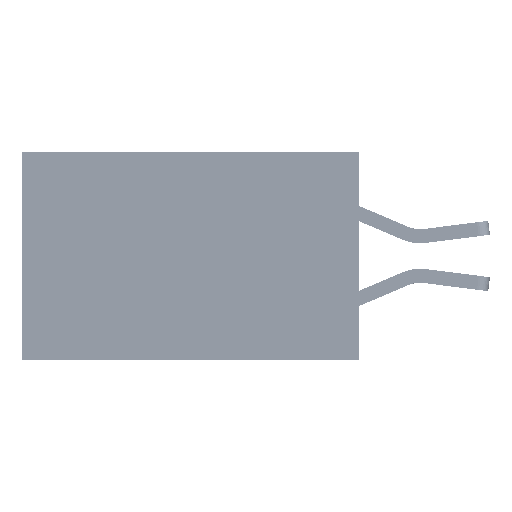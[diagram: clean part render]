
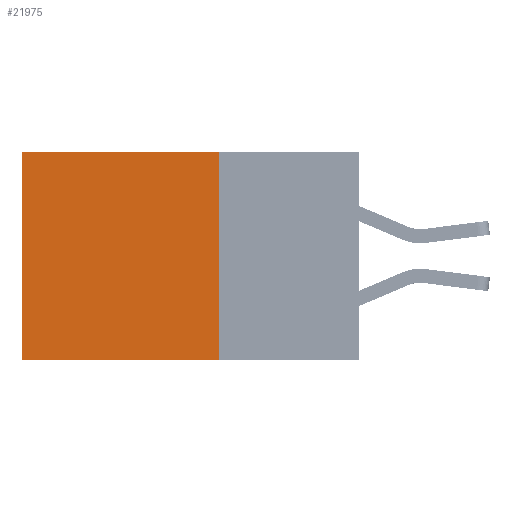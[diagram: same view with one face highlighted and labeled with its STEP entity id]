
A CAD part, left-side view. The second image highlights one B-rep face of the part: STEP entity #21975.
In plain terms, the highlighted planar face has unit normal (-1, 0, 0).
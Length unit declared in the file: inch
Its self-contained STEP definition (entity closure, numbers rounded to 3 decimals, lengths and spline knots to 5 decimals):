
#781 = DIRECTION ( 'NONE',  ( 0., 0., -1. ) ) ;
#990 = CARTESIAN_POINT ( 'NONE',  ( 0.2875, 0.25, -0.37 ) ) ;
#1263 = PLANE ( 'NONE',  #16572 ) ;
#1354 = ORIENTED_EDGE ( 'NONE', *, *, #22394, .T. ) ;
#1363 = LINE ( 'NONE', #17953, #22209 ) ;
#2689 = VERTEX_POINT ( 'NONE', #40871 ) ;
#2966 = DIRECTION ( 'NONE',  ( 0., 0., -1. ) ) ;
#4095 = ORIENTED_EDGE ( 'NONE', *, *, #32219, .T. ) ;
#7632 = CARTESIAN_POINT ( 'NONE',  ( 0.2875, 0.25, 0. ) ) ;
#13044 = ORIENTED_EDGE ( 'NONE', *, *, #46236, .F. ) ;
#14273 = CARTESIAN_POINT ( 'NONE',  ( 0.2875, 0.25, -0.37 ) ) ;
#15764 = CARTESIAN_POINT ( 'NONE',  ( 0.2875, 0.25, 0. ) ) ;
#16572 = AXIS2_PLACEMENT_3D ( 'NONE', #15764, #19606, #781 ) ;
#16774 = VECTOR ( 'NONE', #41909, 39.37008 ) ;
#17953 = CARTESIAN_POINT ( 'NONE',  ( 0.2875, 0.6, 0. ) ) ;
#18888 = CARTESIAN_POINT ( 'NONE',  ( 0.2875, 0.25, 0. ) ) ;
#19161 = ORIENTED_EDGE ( 'NONE', *, *, #20417, .F. ) ;
#19606 = DIRECTION ( 'NONE',  ( 1., 0., 0. ) ) ;
#20417 = EDGE_CURVE ( 'NONE', #2689, #37958, #30584, .T. ) ;
#21975 = ADVANCED_FACE ( 'NONE', ( #47173 ), #1263, .F. ) ;
#22209 = VECTOR ( 'NONE', #2966, 39.37008 ) ;
#22394 = EDGE_CURVE ( 'NONE', #2689, #31324, #41734, .T. ) ;
#23217 = LINE ( 'NONE', #990, #31672 ) ;
#26621 = EDGE_LOOP ( 'NONE', ( #4095, #13044, #19161, #1354 ) ) ;
#30584 = LINE ( 'NONE', #7632, #16774 ) ;
#31324 = VERTEX_POINT ( 'NONE', #43432 ) ;
#31359 = VERTEX_POINT ( 'NONE', #35048 ) ;
#31672 = VECTOR ( 'NONE', #39250, 39.37008 ) ;
#32219 = EDGE_CURVE ( 'NONE', #31324, #31359, #1363, .T. ) ;
#35048 = CARTESIAN_POINT ( 'NONE',  ( 0.2875, 0.6, -0.37 ) ) ;
#37958 = VERTEX_POINT ( 'NONE', #14273 ) ;
#39250 = DIRECTION ( 'NONE',  ( 0., 1., 0. ) ) ;
#39336 = VECTOR ( 'NONE', #49417, 39.37008 ) ;
#40871 = CARTESIAN_POINT ( 'NONE',  ( 0.2875, 0.25, 0. ) ) ;
#41734 = LINE ( 'NONE', #18888, #39336 ) ;
#41909 = DIRECTION ( 'NONE',  ( 0., 0., -1. ) ) ;
#43432 = CARTESIAN_POINT ( 'NONE',  ( 0.2875, 0.6, 0. ) ) ;
#46236 = EDGE_CURVE ( 'NONE', #37958, #31359, #23217, .T. ) ;
#47173 = FACE_OUTER_BOUND ( 'NONE', #26621, .T. ) ;
#49417 = DIRECTION ( 'NONE',  ( 0., 1., 0. ) ) ;
